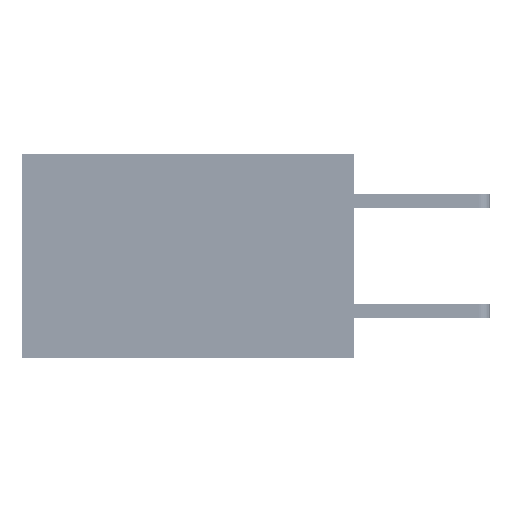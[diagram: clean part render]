
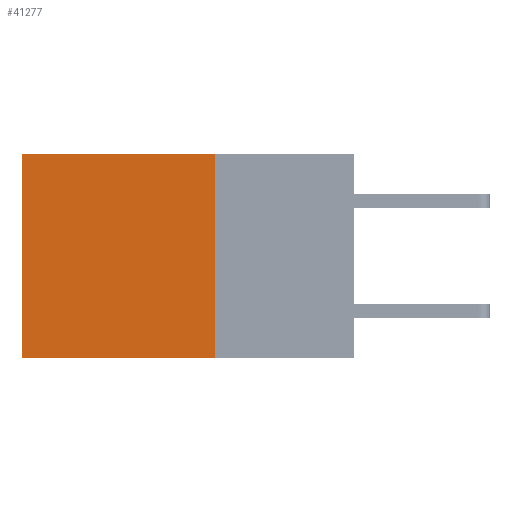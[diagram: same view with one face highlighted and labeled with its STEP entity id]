
A CAD part, left-side view. The second image highlights one B-rep face of the part: STEP entity #41277.
In plain terms, the highlighted planar face has unit normal (-1, 0, 0).
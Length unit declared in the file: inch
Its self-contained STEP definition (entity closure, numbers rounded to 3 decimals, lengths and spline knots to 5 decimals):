
#644 = EDGE_CURVE ( 'NONE', #11379, #7907, #12047, .T. ) ;
#661 = VECTOR ( 'NONE', #36188, 39.37008 ) ;
#1168 = VERTEX_POINT ( 'NONE', #22555 ) ;
#1996 = DIRECTION ( 'NONE',  ( 0., 0., -1. ) ) ;
#4587 = CARTESIAN_POINT ( 'NONE',  ( 0.2875, 0.25, 0. ) ) ;
#5312 = ORIENTED_EDGE ( 'NONE', *, *, #23406, .F. ) ;
#5990 = CARTESIAN_POINT ( 'NONE',  ( 0.2875, 0.25, 0. ) ) ;
#7907 = VERTEX_POINT ( 'NONE', #8428 ) ;
#8428 = CARTESIAN_POINT ( 'NONE',  ( 0.2875, 0.6, 0. ) ) ;
#8655 = EDGE_LOOP ( 'NONE', ( #12208, #5312, #24705, #23417 ) ) ;
#9734 = EDGE_CURVE ( 'NONE', #11379, #1168, #25443, .T. ) ;
#11379 = VERTEX_POINT ( 'NONE', #4587 ) ;
#12047 = LINE ( 'NONE', #5990, #661 ) ;
#12208 = ORIENTED_EDGE ( 'NONE', *, *, #23816, .T. ) ;
#12951 = CARTESIAN_POINT ( 'NONE',  ( 0.2875, 0.25, -0.37 ) ) ;
#14921 = PLANE ( 'NONE',  #28231 ) ;
#15146 = VECTOR ( 'NONE', #32807, 39.37008 ) ;
#15177 = VECTOR ( 'NONE', #1996, 39.37008 ) ;
#16274 = CARTESIAN_POINT ( 'NONE',  ( 0.2875, 0.6, -0.37 ) ) ;
#18231 = DIRECTION ( 'NONE',  ( 1., 0., 0. ) ) ;
#22224 = VERTEX_POINT ( 'NONE', #16274 ) ;
#22555 = CARTESIAN_POINT ( 'NONE',  ( 0.2875, 0.25, -0.37 ) ) ;
#23341 = VECTOR ( 'NONE', #24906, 39.37008 ) ;
#23406 = EDGE_CURVE ( 'NONE', #1168, #22224, #26985, .T. ) ;
#23417 = ORIENTED_EDGE ( 'NONE', *, *, #644, .T. ) ;
#23816 = EDGE_CURVE ( 'NONE', #7907, #22224, #35158, .T. ) ;
#24705 = ORIENTED_EDGE ( 'NONE', *, *, #9734, .F. ) ;
#24906 = DIRECTION ( 'NONE',  ( 0., 0., -1. ) ) ;
#25443 = LINE ( 'NONE', #41321, #15177 ) ;
#26985 = LINE ( 'NONE', #12951, #15146 ) ;
#28231 = AXIS2_PLACEMENT_3D ( 'NONE', #37884, #18231, #41205 ) ;
#32807 = DIRECTION ( 'NONE',  ( 0., 1., 0. ) ) ;
#34648 = CARTESIAN_POINT ( 'NONE',  ( 0.2875, 0.6, 0. ) ) ;
#35158 = LINE ( 'NONE', #34648, #23341 ) ;
#36188 = DIRECTION ( 'NONE',  ( 0., 1., 0. ) ) ;
#37884 = CARTESIAN_POINT ( 'NONE',  ( 0.2875, 0.25, 0. ) ) ;
#39080 = FACE_OUTER_BOUND ( 'NONE', #8655, .T. ) ;
#41205 = DIRECTION ( 'NONE',  ( 0., 0., -1. ) ) ;
#41277 = ADVANCED_FACE ( 'NONE', ( #39080 ), #14921, .F. ) ;
#41321 = CARTESIAN_POINT ( 'NONE',  ( 0.2875, 0.25, 0. ) ) ;
